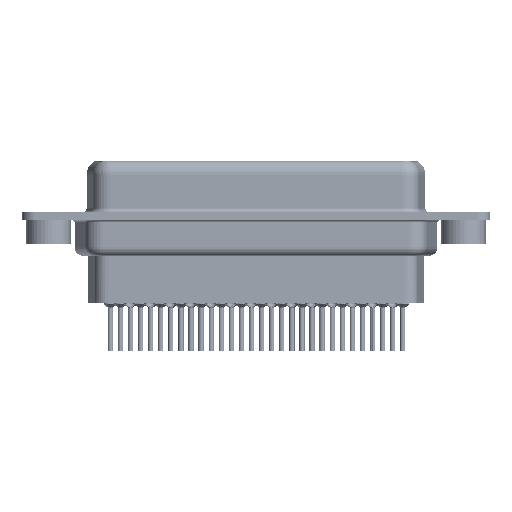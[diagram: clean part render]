
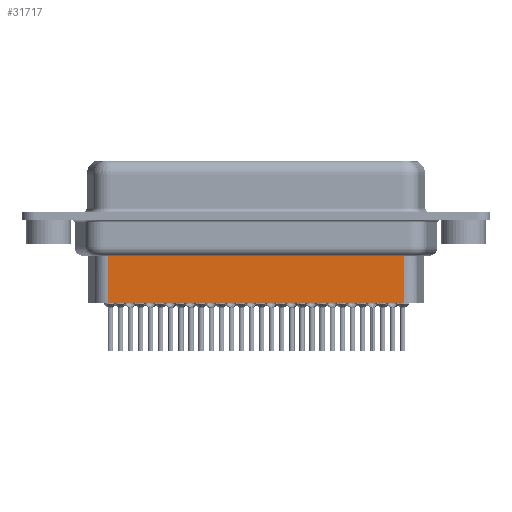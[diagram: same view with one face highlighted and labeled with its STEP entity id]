
A CAD part, front view. The second image highlights one B-rep face of the part: STEP entity #31717.
In plain terms, the highlighted planar face has unit normal (0, -1, 0).
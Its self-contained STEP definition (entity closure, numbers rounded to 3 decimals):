
#1237 = ORIENTED_EDGE ( 'NONE', *, *, #2132, .F. ) ;
#2132 = EDGE_CURVE ( 'NONE', #20386, #21409, #27690, .T. ) ;
#2479 = DIRECTION ( 'NONE',  ( -1., 0., 0. ) ) ;
#5700 = ORIENTED_EDGE ( 'NONE', *, *, #12117, .F. ) ;
#8513 = EDGE_LOOP ( 'NONE', ( #1237, #10313, #18819, #5700 ) ) ;
#9188 = FACE_OUTER_BOUND ( 'NONE', #8513, .T. ) ;
#9543 = DIRECTION ( 'NONE',  ( 0., 0., -1. ) ) ;
#10078 = EDGE_CURVE ( 'NONE', #20386, #32011, #39190, .T. ) ;
#10313 = ORIENTED_EDGE ( 'NONE', *, *, #10078, .T. ) ;
#10724 = LINE ( 'NONE', #20006, #14326 ) ;
#12117 = EDGE_CURVE ( 'NONE', #21409, #30118, #10724, .T. ) ;
#12371 = CARTESIAN_POINT ( 'NONE',  ( 40.339, -3.5, -3.1 ) ) ;
#13144 = CARTESIAN_POINT ( 'NONE',  ( 40.339, -3.5, -9.85 ) ) ;
#13883 = VECTOR ( 'NONE', #2479, 1000. ) ;
#14326 = VECTOR ( 'NONE', #32504, 1000. ) ;
#14808 = CARTESIAN_POINT ( 'NONE',  ( 40.339, -3.5, -4.097 ) ) ;
#17059 = CARTESIAN_POINT ( 'NONE',  ( 6.701, -3.5, -3.1 ) ) ;
#18460 = DIRECTION ( 'NONE',  ( 1., 0., 0. ) ) ;
#18819 = ORIENTED_EDGE ( 'NONE', *, *, #31452, .T. ) ;
#19896 = LINE ( 'NONE', #17059, #22340 ) ;
#20006 = CARTESIAN_POINT ( 'NONE',  ( 6.701, -3.5, -9.85 ) ) ;
#20386 = VERTEX_POINT ( 'NONE', #14808 ) ;
#21141 = CARTESIAN_POINT ( 'NONE',  ( 6.701, -3.5, -9.85 ) ) ;
#21409 = VERTEX_POINT ( 'NONE', #13144 ) ;
#22340 = VECTOR ( 'NONE', #32192, 1000. ) ;
#27690 = LINE ( 'NONE', #12371, #27775 ) ;
#27692 = CARTESIAN_POINT ( 'NONE',  ( 6.701, -3.5, -4.097 ) ) ;
#27775 = VECTOR ( 'NONE', #9543, 1000. ) ;
#30044 = AXIS2_PLACEMENT_3D ( 'NONE', #33989, #33786, #18460 ) ;
#30114 = CARTESIAN_POINT ( 'NONE',  ( 6.454, -3.5, -4.097 ) ) ;
#30118 = VERTEX_POINT ( 'NONE', #21141 ) ;
#31452 = EDGE_CURVE ( 'NONE', #32011, #30118, #19896, .T. ) ;
#31717 = ADVANCED_FACE ( 'NONE', ( #9188 ), #36998, .T. ) ;
#32011 = VERTEX_POINT ( 'NONE', #27692 ) ;
#32192 = DIRECTION ( 'NONE',  ( 0., 0., -1. ) ) ;
#32504 = DIRECTION ( 'NONE',  ( -1., 0., 0. ) ) ;
#33786 = DIRECTION ( 'NONE',  ( 0., -1., 0. ) ) ;
#33989 = CARTESIAN_POINT ( 'NONE',  ( 6.701, -3.5, -3.1 ) ) ;
#36998 = PLANE ( 'NONE',  #30044 ) ;
#39190 = LINE ( 'NONE', #30114, #13883 ) ;
